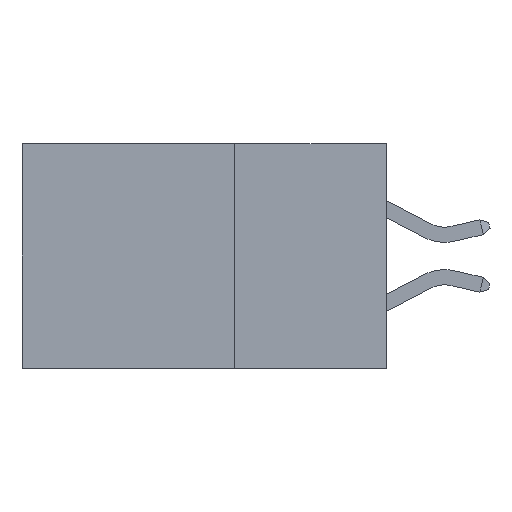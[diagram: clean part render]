
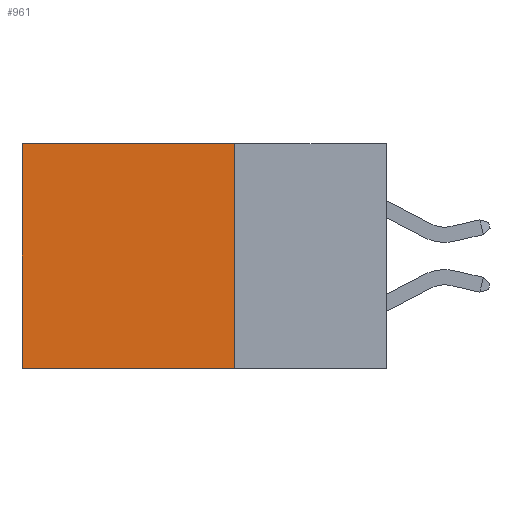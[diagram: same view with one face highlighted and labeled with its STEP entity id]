
A CAD part, left-side view. The second image highlights one B-rep face of the part: STEP entity #961.
In plain terms, the highlighted planar face has unit normal (-1, 0, 0).
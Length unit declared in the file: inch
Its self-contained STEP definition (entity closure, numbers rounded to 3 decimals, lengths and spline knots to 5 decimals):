
#204 = VERTEX_POINT ( 'NONE', #11622 ) ;
#839 = DIRECTION ( 'NONE',  ( 0., 1., 0. ) ) ;
#961 = ADVANCED_FACE ( 'NONE', ( #2616 ), #16157, .F. ) ;
#1194 = LINE ( 'NONE', #7066, #7592 ) ;
#1448 = DIRECTION ( 'NONE',  ( 0., 0., -1. ) ) ;
#2410 = ORIENTED_EDGE ( 'NONE', *, *, #9210, .F. ) ;
#2420 = CARTESIAN_POINT ( 'NONE',  ( 0.298, 0.6, 0. ) ) ;
#2616 = FACE_OUTER_BOUND ( 'NONE', #10309, .T. ) ;
#3007 = ORIENTED_EDGE ( 'NONE', *, *, #9028, .F. ) ;
#3208 = VECTOR ( 'NONE', #13204, 39.37008 ) ;
#4465 = AXIS2_PLACEMENT_3D ( 'NONE', #16509, #16289, #1448 ) ;
#4504 = VERTEX_POINT ( 'NONE', #15789 ) ;
#5500 = DIRECTION ( 'NONE',  ( 0., 0., -1. ) ) ;
#5614 = LINE ( 'NONE', #13209, #11680 ) ;
#6913 = VERTEX_POINT ( 'NONE', #8969 ) ;
#7066 = CARTESIAN_POINT ( 'NONE',  ( 0.298, 0.25, 0. ) ) ;
#7351 = EDGE_CURVE ( 'NONE', #4504, #14957, #11922, .T. ) ;
#7592 = VECTOR ( 'NONE', #14749, 39.37008 ) ;
#8165 = ORIENTED_EDGE ( 'NONE', *, *, #8472, .T. ) ;
#8446 = VECTOR ( 'NONE', #839, 39.37008 ) ;
#8472 = EDGE_CURVE ( 'NONE', #14957, #204, #5614, .T. ) ;
#8969 = CARTESIAN_POINT ( 'NONE',  ( 0.298, 0.25, -0.37 ) ) ;
#9028 = EDGE_CURVE ( 'NONE', #6913, #204, #10023, .T. ) ;
#9210 = EDGE_CURVE ( 'NONE', #4504, #6913, #1194, .T. ) ;
#10023 = LINE ( 'NONE', #11942, #3208 ) ;
#10309 = EDGE_LOOP ( 'NONE', ( #8165, #3007, #2410, #12607 ) ) ;
#11622 = CARTESIAN_POINT ( 'NONE',  ( 0.298, 0.6, -0.37 ) ) ;
#11680 = VECTOR ( 'NONE', #5500, 39.37008 ) ;
#11922 = LINE ( 'NONE', #16191, #8446 ) ;
#11942 = CARTESIAN_POINT ( 'NONE',  ( 0.298, 0.25, -0.37 ) ) ;
#12607 = ORIENTED_EDGE ( 'NONE', *, *, #7351, .T. ) ;
#13204 = DIRECTION ( 'NONE',  ( 0., 1., 0. ) ) ;
#13209 = CARTESIAN_POINT ( 'NONE',  ( 0.298, 0.6, 0. ) ) ;
#14749 = DIRECTION ( 'NONE',  ( 0., 0., -1. ) ) ;
#14957 = VERTEX_POINT ( 'NONE', #2420 ) ;
#15789 = CARTESIAN_POINT ( 'NONE',  ( 0.298, 0.25, 0. ) ) ;
#16157 = PLANE ( 'NONE',  #4465 ) ;
#16191 = CARTESIAN_POINT ( 'NONE',  ( 0.298, 0.25, 0. ) ) ;
#16289 = DIRECTION ( 'NONE',  ( 1., 0., 0. ) ) ;
#16509 = CARTESIAN_POINT ( 'NONE',  ( 0.298, 0.25, 0. ) ) ;
